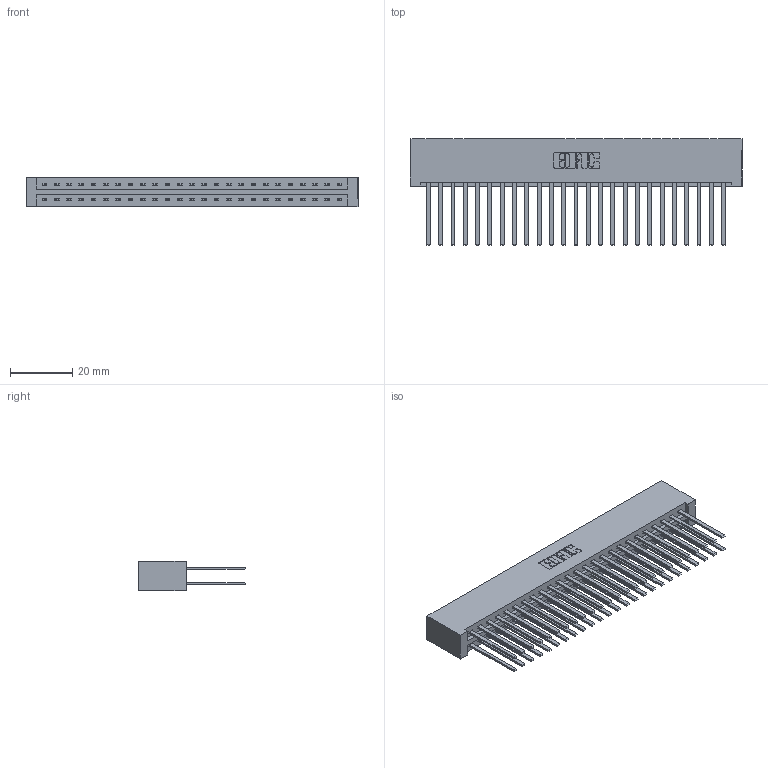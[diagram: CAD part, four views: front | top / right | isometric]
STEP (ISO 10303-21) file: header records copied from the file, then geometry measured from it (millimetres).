
FILE_DESCRIPTION (( 'STEP AP203' ), '1' );
FILE_NAME ('337-050-544-201.STEP', '2019-10-09T15:58:00', ( '' ), ( '' ), 'SwSTEP 2.0', 'SolidWorks 2016', '' );
FILE_SCHEMA (( 'CONFIG_CONTROL_DESIGN' ));
Length unit declared in the file: inch
Products named in the file (3): 337 Part_No Mounting Lugs; 337-050-544-201; 345-292-001_345-293-144
Assembly tree (51 placements, depth 2):
  337-050-544-201
    337 Part_No Mounting Lugs
    345-292-001_345-293-144  x50
Bounding box: 106.93 x 34.3 x 9.4 mm (x, y, z)
Volume: 12504.9 mm3; surface area: 16317.5 mm2
Topology: 51 solids, 51 shells, 2506 faces, 7437 edges, 4890 vertices
Faces by surface type: plane 1766, cylinder 740
Entity records: 21121 total; most frequent: CARTESIAN_POINT 3570, ORIENTED_EDGE 3506, DIRECTION 3057, EDGE_CURVE 1753, VECTOR 1637, LINE 1637, VERTEX_POINT 1166, AXIS2_PLACEMENT_3D 710
